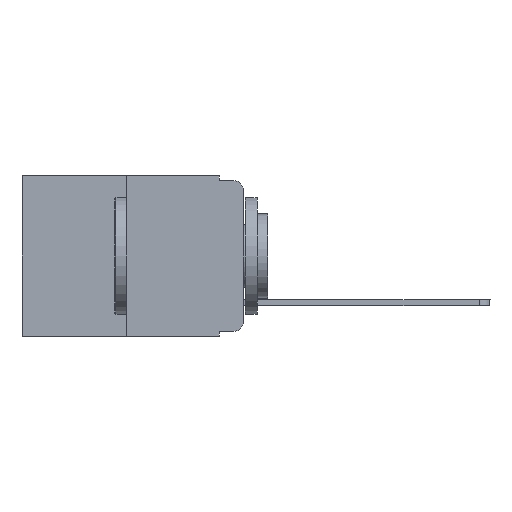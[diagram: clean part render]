
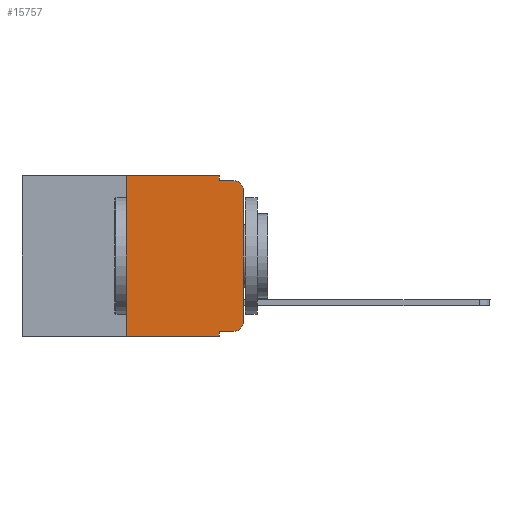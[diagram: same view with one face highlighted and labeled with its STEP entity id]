
A CAD part, left-side view. The second image highlights one B-rep face of the part: STEP entity #15757.
In plain terms, the highlighted planar face has unit normal (-1, 0, 0).
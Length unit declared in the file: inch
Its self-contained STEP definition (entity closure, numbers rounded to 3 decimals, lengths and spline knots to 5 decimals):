
#96 = LINE ( 'NONE', #2246, #10483 ) ;
#254 = CARTESIAN_POINT ( 'NONE',  ( 0., 0.25, 0. ) ) ;
#359 = VERTEX_POINT ( 'NONE', #4966 ) ;
#441 = CARTESIAN_POINT ( 'NONE',  ( 0., 0.25, -0.343 ) ) ;
#622 = PLANE ( 'NONE',  #12116 ) ;
#941 = CARTESIAN_POINT ( 'NONE',  ( 0., 0.02, -0.313 ) ) ;
#1099 = LINE ( 'NONE', #254, #17152 ) ;
#1153 = EDGE_CURVE ( 'NONE', #359, #9844, #8886, .T. ) ;
#1378 = LINE ( 'NONE', #7697, #10039 ) ;
#1547 = CARTESIAN_POINT ( 'NONE',  ( 0., 0.051, 0. ) ) ;
#1739 = CARTESIAN_POINT ( 'NONE',  ( 0., 0.051, 0. ) ) ;
#1814 = EDGE_CURVE ( 'NONE', #3043, #2291, #8415, .T. ) ;
#2175 = VECTOR ( 'NONE', #17033, 39.37008 ) ;
#2246 = CARTESIAN_POINT ( 'NONE',  ( 0., 0.051, -0.333 ) ) ;
#2291 = VERTEX_POINT ( 'NONE', #5613 ) ;
#2395 = EDGE_CURVE ( 'NONE', #16308, #7611, #1099, .T. ) ;
#2584 = CARTESIAN_POINT ( 'NONE',  ( 0., 0.02, -0.01 ) ) ;
#2641 = CARTESIAN_POINT ( 'NONE',  ( 0., 0.02, -0.333 ) ) ;
#2847 = VECTOR ( 'NONE', #4850, 39.37008 ) ;
#3043 = VERTEX_POINT ( 'NONE', #3045 ) ;
#3045 = CARTESIAN_POINT ( 'NONE',  ( 0., 0.051, 0. ) ) ;
#3152 = DIRECTION ( 'NONE',  ( 0., 0., 1. ) ) ;
#3398 = DIRECTION ( 'NONE',  ( 0., -1., 0. ) ) ;
#3406 = DIRECTION ( 'NONE',  ( 0., 0., -1. ) ) ;
#3543 = CARTESIAN_POINT ( 'NONE',  ( 0., 0., 0. ) ) ;
#4030 = LINE ( 'NONE', #6923, #9442 ) ;
#4099 = CARTESIAN_POINT ( 'NONE',  ( 0., 0.051, -0.333 ) ) ;
#4414 = FACE_OUTER_BOUND ( 'NONE', #5341, .T. ) ;
#4818 = CARTESIAN_POINT ( 'NONE',  ( 0., 0.02, -0.03 ) ) ;
#4850 = DIRECTION ( 'NONE',  ( 0., 0., 1. ) ) ;
#4872 = EDGE_CURVE ( 'NONE', #9844, #13554, #17047, .T. ) ;
#4935 = ORIENTED_EDGE ( 'NONE', *, *, #16694, .T. ) ;
#4966 = CARTESIAN_POINT ( 'NONE',  ( 0., 0., -0.313 ) ) ;
#5341 = EDGE_LOOP ( 'NONE', ( #14742, #8862, #9982, #7977, #11719, #15675, #9971, #7586, #9219, #4935 ) ) ;
#5613 = CARTESIAN_POINT ( 'NONE',  ( 0., 0.051, -0.01 ) ) ;
#5966 = EDGE_CURVE ( 'NONE', #7611, #3043, #1378, .T. ) ;
#6590 = DIRECTION ( 'NONE',  ( 0., 0., -1. ) ) ;
#6681 = VECTOR ( 'NONE', #11413, 39.37008 ) ;
#6842 = CARTESIAN_POINT ( 'NONE',  ( 0., 0.25, 0. ) ) ;
#6923 = CARTESIAN_POINT ( 'NONE',  ( 0., 0.051, -0.01 ) ) ;
#6981 = AXIS2_PLACEMENT_3D ( 'NONE', #941, #13669, #6590 ) ;
#7586 = ORIENTED_EDGE ( 'NONE', *, *, #11914, .F. ) ;
#7611 = VERTEX_POINT ( 'NONE', #6842 ) ;
#7683 = VERTEX_POINT ( 'NONE', #4099 ) ;
#7697 = CARTESIAN_POINT ( 'NONE',  ( 0., 0.473, 0. ) ) ;
#7733 = CARTESIAN_POINT ( 'NONE',  ( 0., 0.473, 0. ) ) ;
#7977 = ORIENTED_EDGE ( 'NONE', *, *, #1814, .F. ) ;
#8415 = LINE ( 'NONE', #1739, #6681 ) ;
#8862 = ORIENTED_EDGE ( 'NONE', *, *, #4872, .T. ) ;
#8886 = LINE ( 'NONE', #3543, #2847 ) ;
#9219 = ORIENTED_EDGE ( 'NONE', *, *, #10843, .T. ) ;
#9435 = EDGE_CURVE ( 'NONE', #2291, #13554, #4030, .T. ) ;
#9442 = VECTOR ( 'NONE', #11014, 39.37008 ) ;
#9844 = VERTEX_POINT ( 'NONE', #15450 ) ;
#9971 = ORIENTED_EDGE ( 'NONE', *, *, #17496, .T. ) ;
#9982 = ORIENTED_EDGE ( 'NONE', *, *, #9435, .F. ) ;
#9985 = CARTESIAN_POINT ( 'NONE',  ( 0., 0.473, -0.343 ) ) ;
#10039 = VECTOR ( 'NONE', #16535, 39.37008 ) ;
#10226 = LINE ( 'NONE', #1547, #12857 ) ;
#10342 = DIRECTION ( 'NONE',  ( 1., 0., 0. ) ) ;
#10483 = VECTOR ( 'NONE', #3398, 39.37008 ) ;
#10507 = DIRECTION ( 'NONE',  ( -1., 0., 0. ) ) ;
#10752 = VERTEX_POINT ( 'NONE', #15656 ) ;
#10843 = EDGE_CURVE ( 'NONE', #7683, #16850, #96, .T. ) ;
#11014 = DIRECTION ( 'NONE',  ( 0., -1., 0. ) ) ;
#11413 = DIRECTION ( 'NONE',  ( 0., 0., -1. ) ) ;
#11719 = ORIENTED_EDGE ( 'NONE', *, *, #5966, .F. ) ;
#11900 = LINE ( 'NONE', #9985, #2175 ) ;
#11914 = EDGE_CURVE ( 'NONE', #7683, #10752, #10226, .T. ) ;
#12116 = AXIS2_PLACEMENT_3D ( 'NONE', #7733, #10342, #3406 ) ;
#12857 = VECTOR ( 'NONE', #12862, 39.37008 ) ;
#12862 = DIRECTION ( 'NONE',  ( 0., 0., -1. ) ) ;
#13182 = AXIS2_PLACEMENT_3D ( 'NONE', #4818, #10507, #17346 ) ;
#13554 = VERTEX_POINT ( 'NONE', #2584 ) ;
#13669 = DIRECTION ( 'NONE',  ( -1., 0., 0. ) ) ;
#14742 = ORIENTED_EDGE ( 'NONE', *, *, #1153, .T. ) ;
#15450 = CARTESIAN_POINT ( 'NONE',  ( 0., 0., -0.03 ) ) ;
#15455 = CIRCLE ( 'NONE', #6981, 0.02 ) ;
#15656 = CARTESIAN_POINT ( 'NONE',  ( 0., 0.051, -0.343 ) ) ;
#15675 = ORIENTED_EDGE ( 'NONE', *, *, #2395, .F. ) ;
#15757 = ADVANCED_FACE ( 'NONE', ( #4414 ), #622, .F. ) ;
#16308 = VERTEX_POINT ( 'NONE', #441 ) ;
#16535 = DIRECTION ( 'NONE',  ( 0., -1., 0. ) ) ;
#16694 = EDGE_CURVE ( 'NONE', #16850, #359, #15455, .T. ) ;
#16850 = VERTEX_POINT ( 'NONE', #2641 ) ;
#17033 = DIRECTION ( 'NONE',  ( 0., -1., 0. ) ) ;
#17047 = CIRCLE ( 'NONE', #13182, 0.02 ) ;
#17152 = VECTOR ( 'NONE', #3152, 39.37008 ) ;
#17346 = DIRECTION ( 'NONE',  ( 0., 0., -1. ) ) ;
#17496 = EDGE_CURVE ( 'NONE', #16308, #10752, #11900, .T. ) ;
